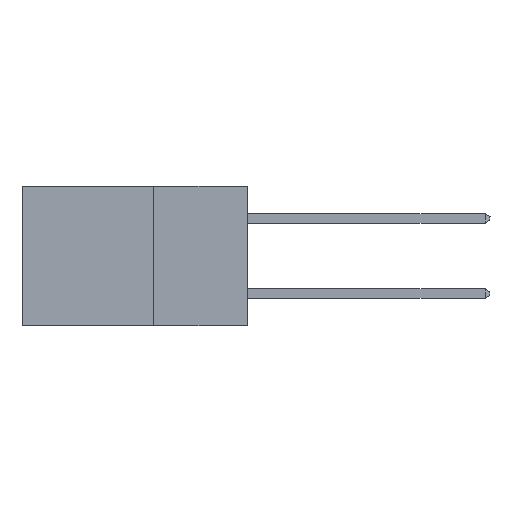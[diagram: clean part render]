
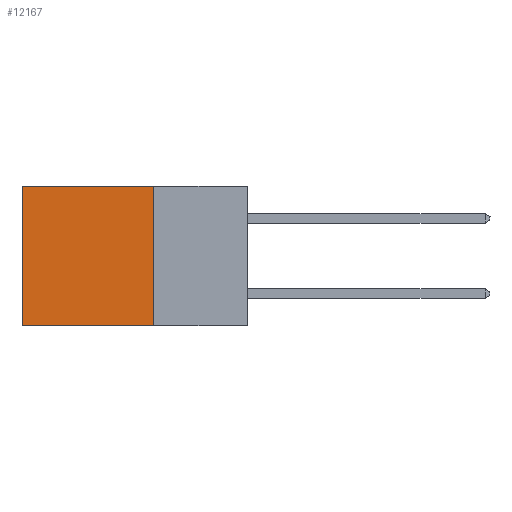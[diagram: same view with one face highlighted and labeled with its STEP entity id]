
A CAD part, left-side view. The second image highlights one B-rep face of the part: STEP entity #12167.
In plain terms, the highlighted planar face has unit normal (-1, 0, 0).
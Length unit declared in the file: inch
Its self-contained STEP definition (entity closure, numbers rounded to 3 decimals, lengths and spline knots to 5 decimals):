
#290 = DIRECTION ( 'NONE',  ( 0., 0., -1. ) ) ;
#916 = CARTESIAN_POINT ( 'NONE',  ( 0.2615, 0.6, 0. ) ) ;
#1100 = EDGE_CURVE ( 'NONE', #11331, #3197, #9652, .T. ) ;
#1475 = DIRECTION ( 'NONE',  ( 1., 0., 0. ) ) ;
#2397 = FACE_OUTER_BOUND ( 'NONE', #14257, .T. ) ;
#2832 = CARTESIAN_POINT ( 'NONE',  ( 0.2615, 0.25, -0.37 ) ) ;
#3197 = VERTEX_POINT ( 'NONE', #2832 ) ;
#3667 = VECTOR ( 'NONE', #8931, 39.37008 ) ;
#3736 = AXIS2_PLACEMENT_3D ( 'NONE', #9756, #1475, #12983 ) ;
#3794 = VECTOR ( 'NONE', #13121, 39.37008 ) ;
#4017 = CARTESIAN_POINT ( 'NONE',  ( 0.2615, 0.25, -0.37 ) ) ;
#4309 = CARTESIAN_POINT ( 'NONE',  ( 0.2615, 0.25, 0. ) ) ;
#4897 = ORIENTED_EDGE ( 'NONE', *, *, #1100, .F. ) ;
#5243 = CARTESIAN_POINT ( 'NONE',  ( 0.2615, 0.25, -0.37 ) ) ;
#6071 = DIRECTION ( 'NONE',  ( 0., 0., -1. ) ) ;
#6159 = ORIENTED_EDGE ( 'NONE', *, *, #6795, .T. ) ;
#6197 = LINE ( 'NONE', #11959, #3794 ) ;
#6438 = EDGE_CURVE ( 'NONE', #3197, #12001, #14845, .T. ) ;
#6766 = CARTESIAN_POINT ( 'NONE',  ( 0.2615, 0.6, -0.37 ) ) ;
#6795 = EDGE_CURVE ( 'NONE', #7512, #12001, #8530, .T. ) ;
#7512 = VERTEX_POINT ( 'NONE', #916 ) ;
#8295 = CARTESIAN_POINT ( 'NONE',  ( 0.2615, 0.6, -0.37 ) ) ;
#8530 = LINE ( 'NONE', #8295, #12759 ) ;
#8931 = DIRECTION ( 'NONE',  ( 0., 1., 0. ) ) ;
#9559 = ORIENTED_EDGE ( 'NONE', *, *, #14596, .T. ) ;
#9652 = LINE ( 'NONE', #4017, #11526 ) ;
#9747 = ORIENTED_EDGE ( 'NONE', *, *, #6438, .F. ) ;
#9756 = CARTESIAN_POINT ( 'NONE',  ( 0.2615, 0.25, -0.37 ) ) ;
#11331 = VERTEX_POINT ( 'NONE', #4309 ) ;
#11526 = VECTOR ( 'NONE', #290, 39.37008 ) ;
#11829 = PLANE ( 'NONE',  #3736 ) ;
#11959 = CARTESIAN_POINT ( 'NONE',  ( 0.2615, 0.25, 0. ) ) ;
#12001 = VERTEX_POINT ( 'NONE', #6766 ) ;
#12167 = ADVANCED_FACE ( 'NONE', ( #2397 ), #11829, .F. ) ;
#12759 = VECTOR ( 'NONE', #6071, 39.37008 ) ;
#12983 = DIRECTION ( 'NONE',  ( 0., 0., -1. ) ) ;
#13121 = DIRECTION ( 'NONE',  ( 0., 1., 0. ) ) ;
#14257 = EDGE_LOOP ( 'NONE', ( #6159, #9747, #4897, #9559 ) ) ;
#14596 = EDGE_CURVE ( 'NONE', #11331, #7512, #6197, .T. ) ;
#14845 = LINE ( 'NONE', #5243, #3667 ) ;
